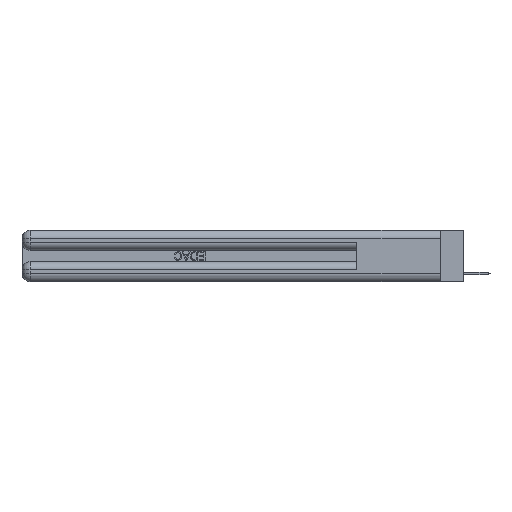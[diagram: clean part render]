
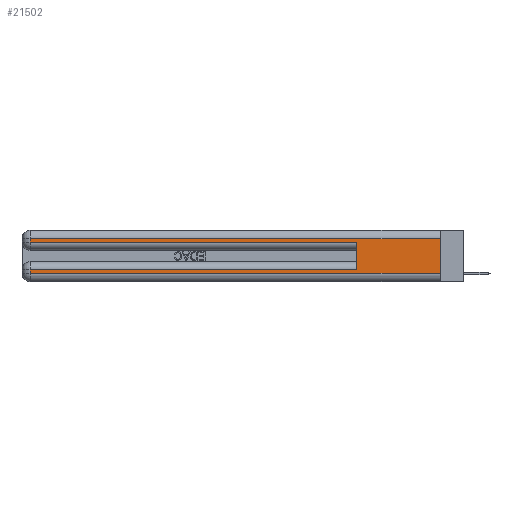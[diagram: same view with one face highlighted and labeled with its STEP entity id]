
A CAD part, left-side view. The second image highlights one B-rep face of the part: STEP entity #21502.
In plain terms, the highlighted planar face has unit normal (-1, 0, 0).
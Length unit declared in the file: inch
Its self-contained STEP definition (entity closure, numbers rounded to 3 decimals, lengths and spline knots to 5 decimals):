
#35 = EDGE_CURVE ( 'NONE', #30265, #14849, #23945, .T. ) ;
#1175 = LINE ( 'NONE', #13631, #2813 ) ;
#1859 = DIRECTION ( 'NONE',  ( 0., 0., -1. ) ) ;
#2175 = DIRECTION ( 'NONE',  ( 0., -1., 0. ) ) ;
#2345 = CARTESIAN_POINT ( 'NONE',  ( 0., 2.94, 0.06 ) ) ;
#2813 = VECTOR ( 'NONE', #31376, 39.37008 ) ;
#2860 = CARTESIAN_POINT ( 'NONE',  ( 0., 0.6, 0.085 ) ) ;
#2876 = ORIENTED_EDGE ( 'NONE', *, *, #14257, .T. ) ;
#3785 = PLANE ( 'NONE',  #22412 ) ;
#3916 = DIRECTION ( 'NONE',  ( 0., 0., -1. ) ) ;
#4557 = EDGE_LOOP ( 'NONE', ( #9827, #25371, #2876, #7106, #23791, #27558, #25245, #26237 ) ) ;
#4683 = VERTEX_POINT ( 'NONE', #5781 ) ;
#5781 = CARTESIAN_POINT ( 'NONE',  ( 0., 2.94, 0.31 ) ) ;
#6308 = CARTESIAN_POINT ( 'NONE',  ( 0., 0., 0.285 ) ) ;
#6555 = VECTOR ( 'NONE', #30239, 39.37008 ) ;
#6720 = CARTESIAN_POINT ( 'NONE',  ( 0., 2.94, 0.37 ) ) ;
#7106 = ORIENTED_EDGE ( 'NONE', *, *, #35, .T. ) ;
#7905 = VECTOR ( 'NONE', #3916, 39.37008 ) ;
#9573 = EDGE_CURVE ( 'NONE', #31227, #13188, #21170, .T. ) ;
#9827 = ORIENTED_EDGE ( 'NONE', *, *, #9573, .F. ) ;
#10140 = CARTESIAN_POINT ( 'NONE',  ( 0., 0., 0.31 ) ) ;
#10633 = CARTESIAN_POINT ( 'NONE',  ( 0., 2.94, 0.085 ) ) ;
#10674 = LINE ( 'NONE', #26684, #7905 ) ;
#10936 = LINE ( 'NONE', #16837, #6555 ) ;
#11305 = EDGE_CURVE ( 'NONE', #31227, #4683, #1175, .T. ) ;
#12649 = EDGE_CURVE ( 'NONE', #16575, #25565, #10674, .T. ) ;
#13188 = VERTEX_POINT ( 'NONE', #32787 ) ;
#13452 = DIRECTION ( 'NONE',  ( 0., -1., 0. ) ) ;
#13631 = CARTESIAN_POINT ( 'NONE',  ( 0., 0., 0.31 ) ) ;
#14257 = EDGE_CURVE ( 'NONE', #4683, #30265, #25966, .T. ) ;
#14849 = VERTEX_POINT ( 'NONE', #32952 ) ;
#16123 = VECTOR ( 'NONE', #24404, 39.37008 ) ;
#16575 = VERTEX_POINT ( 'NONE', #10633 ) ;
#16837 = CARTESIAN_POINT ( 'NONE',  ( 0., 0., 0.085 ) ) ;
#16999 = CARTESIAN_POINT ( 'NONE',  ( 0., 0., 0.06 ) ) ;
#17337 = EDGE_CURVE ( 'NONE', #25565, #13188, #19410, .T. ) ;
#17700 = CARTESIAN_POINT ( 'NONE',  ( 0., 0., 0.37 ) ) ;
#18188 = LINE ( 'NONE', #23397, #19744 ) ;
#18328 = EDGE_CURVE ( 'NONE', #19575, #14849, #18188, .T. ) ;
#18430 = DIRECTION ( 'NONE',  ( 0., 0., 1. ) ) ;
#19410 = LINE ( 'NONE', #16999, #28912 ) ;
#19575 = VERTEX_POINT ( 'NONE', #2860 ) ;
#19744 = VECTOR ( 'NONE', #18430, 39.37008 ) ;
#19978 = EDGE_CURVE ( 'NONE', #19575, #16575, #10936, .T. ) ;
#21170 = LINE ( 'NONE', #17700, #23167 ) ;
#21502 = ADVANCED_FACE ( 'NONE', ( #22662 ), #3785, .F. ) ;
#21922 = CARTESIAN_POINT ( 'NONE',  ( 0., 0., 0.37 ) ) ;
#22412 = AXIS2_PLACEMENT_3D ( 'NONE', #21922, #32216, #1859 ) ;
#22662 = FACE_OUTER_BOUND ( 'NONE', #4557, .T. ) ;
#23167 = VECTOR ( 'NONE', #26051, 39.37008 ) ;
#23397 = CARTESIAN_POINT ( 'NONE',  ( 0., 0.6, 0.145 ) ) ;
#23791 = ORIENTED_EDGE ( 'NONE', *, *, #18328, .F. ) ;
#23945 = LINE ( 'NONE', #6308, #31147 ) ;
#24404 = DIRECTION ( 'NONE',  ( 0., 0., -1. ) ) ;
#25245 = ORIENTED_EDGE ( 'NONE', *, *, #12649, .T. ) ;
#25371 = ORIENTED_EDGE ( 'NONE', *, *, #11305, .T. ) ;
#25565 = VERTEX_POINT ( 'NONE', #2345 ) ;
#25966 = LINE ( 'NONE', #6720, #16123 ) ;
#26051 = DIRECTION ( 'NONE',  ( 0., 0., -1. ) ) ;
#26237 = ORIENTED_EDGE ( 'NONE', *, *, #17337, .T. ) ;
#26684 = CARTESIAN_POINT ( 'NONE',  ( 0., 2.94, 0.37 ) ) ;
#27558 = ORIENTED_EDGE ( 'NONE', *, *, #19978, .T. ) ;
#28912 = VECTOR ( 'NONE', #2175, 39.37008 ) ;
#30239 = DIRECTION ( 'NONE',  ( 0., 1., 0. ) ) ;
#30265 = VERTEX_POINT ( 'NONE', #32704 ) ;
#31147 = VECTOR ( 'NONE', #13452, 39.37008 ) ;
#31227 = VERTEX_POINT ( 'NONE', #10140 ) ;
#31376 = DIRECTION ( 'NONE',  ( 0., 1., 0. ) ) ;
#32216 = DIRECTION ( 'NONE',  ( 1., 0., 0. ) ) ;
#32704 = CARTESIAN_POINT ( 'NONE',  ( 0., 2.94, 0.285 ) ) ;
#32787 = CARTESIAN_POINT ( 'NONE',  ( 0., 0., 0.06 ) ) ;
#32952 = CARTESIAN_POINT ( 'NONE',  ( 0., 0.6, 0.285 ) ) ;
